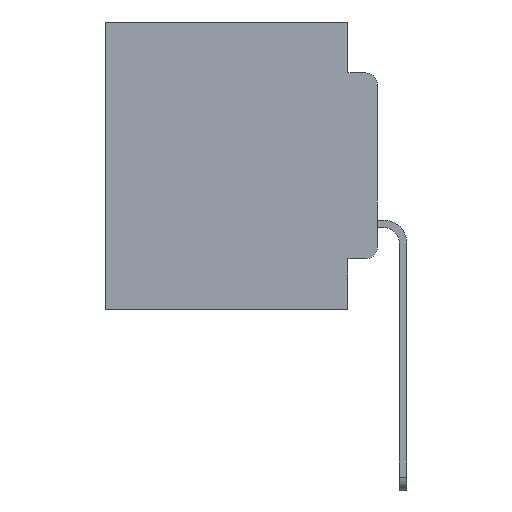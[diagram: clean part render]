
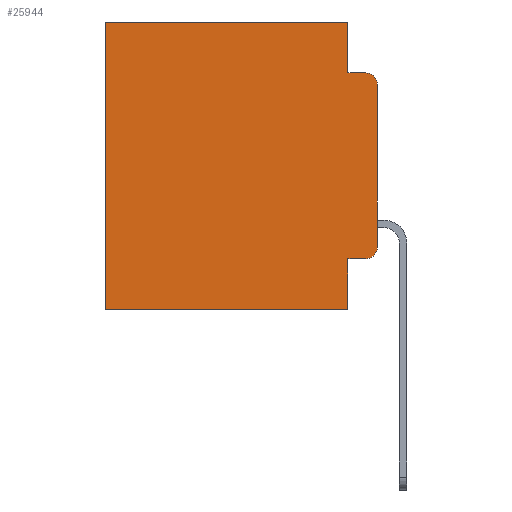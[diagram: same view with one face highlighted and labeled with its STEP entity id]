
A CAD part, left-side view. The second image highlights one B-rep face of the part: STEP entity #25944.
In plain terms, the highlighted planar face has unit normal (-1, 0, 0).
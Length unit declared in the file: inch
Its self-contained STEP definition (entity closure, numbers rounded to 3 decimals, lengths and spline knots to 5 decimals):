
#143 = CARTESIAN_POINT ( 'NONE',  ( 0.298, 0.051, 0. ) ) ;
#675 = EDGE_CURVE ( 'NONE', #21262, #17718, #24937, .T. ) ;
#770 = EDGE_CURVE ( 'NONE', #8905, #21262, #11966, .T. ) ;
#814 = EDGE_CURVE ( 'NONE', #8905, #18406, #3340, .T. ) ;
#872 = EDGE_CURVE ( 'NONE', #12851, #16531, #16743, .T. ) ;
#908 = EDGE_CURVE ( 'NONE', #21166, #15340, #10977, .T. ) ;
#920 = EDGE_CURVE ( 'NONE', #15340, #24086, #20566, .T. ) ;
#952 = EDGE_CURVE ( 'NONE', #9376, #24086, #14355, .T. ) ;
#1000 = EDGE_CURVE ( 'NONE', #9376, #17718, #1510, .T. ) ;
#1510 = LINE ( 'NONE', #13887, #7711 ) ;
#2971 = EDGE_CURVE ( 'NONE', #18406, #16531, #25428, .T. ) ;
#3140 = ORIENTED_EDGE ( 'NONE', *, *, #4649, .T. ) ;
#3340 = LINE ( 'NONE', #143, #10024 ) ;
#4429 = VECTOR ( 'NONE', #13042, 39.37008 ) ;
#4486 = CARTESIAN_POINT ( 'NONE',  ( 0.298, 0.051, -0.0885 ) ) ;
#4649 = EDGE_CURVE ( 'NONE', #21166, #12851, #20337, .T. ) ;
#5161 = AXIS2_PLACEMENT_3D ( 'NONE', #17156, #17014, #17749 ) ;
#5335 = ORIENTED_EDGE ( 'NONE', *, *, #675, .T. ) ;
#6407 = ORIENTED_EDGE ( 'NONE', *, *, #920, .F. ) ;
#6956 = PLANE ( 'NONE',  #23720 ) ;
#7711 = VECTOR ( 'NONE', #15707, 39.37008 ) ;
#8713 = DIRECTION ( 'NONE',  ( 0., 0., -1. ) ) ;
#8905 = VERTEX_POINT ( 'NONE', #20003 ) ;
#8941 = DIRECTION ( 'NONE',  ( 0., -1., 0. ) ) ;
#9144 = DIRECTION ( 'NONE',  ( 0., 0., -1. ) ) ;
#9376 = VERTEX_POINT ( 'NONE', #21919 ) ;
#9735 = CARTESIAN_POINT ( 'NONE',  ( 0.298, 0.473, -0.5 ) ) ;
#9826 = ORIENTED_EDGE ( 'NONE', *, *, #2971, .F. ) ;
#10024 = VECTOR ( 'NONE', #8713, 39.37008 ) ;
#10456 = ORIENTED_EDGE ( 'NONE', *, *, #770, .T. ) ;
#10885 = VECTOR ( 'NONE', #13957, 39.37008 ) ;
#10977 = LINE ( 'NONE', #17508, #25511 ) ;
#11966 = LINE ( 'NONE', #15348, #16449 ) ;
#12851 = VERTEX_POINT ( 'NONE', #17704 ) ;
#13042 = DIRECTION ( 'NONE',  ( 0., -1., 0. ) ) ;
#13094 = CARTESIAN_POINT ( 'NONE',  ( 0.298, 0.051, -0.0885 ) ) ;
#13291 = ORIENTED_EDGE ( 'NONE', *, *, #908, .F. ) ;
#13887 = CARTESIAN_POINT ( 'NONE',  ( 0.298, 0., 0. ) ) ;
#13957 = DIRECTION ( 'NONE',  ( 0., 1., 0. ) ) ;
#14355 = CIRCLE ( 'NONE', #22006, 0.02 ) ;
#15098 = ORIENTED_EDGE ( 'NONE', *, *, #814, .F. ) ;
#15340 = VERTEX_POINT ( 'NONE', #4486 ) ;
#15348 = CARTESIAN_POINT ( 'NONE',  ( 0.298, 0.051, -0.4115 ) ) ;
#15626 = CARTESIAN_POINT ( 'NONE',  ( 0.298, 0.473, 0. ) ) ;
#15707 = DIRECTION ( 'NONE',  ( 0., 0., -1. ) ) ;
#15964 = ORIENTED_EDGE ( 'NONE', *, *, #952, .T. ) ;
#16449 = VECTOR ( 'NONE', #8941, 39.37008 ) ;
#16531 = VERTEX_POINT ( 'NONE', #9735 ) ;
#16598 = DIRECTION ( 'NONE',  ( -1., 0., 0. ) ) ;
#16648 = CARTESIAN_POINT ( 'NONE',  ( 0.298, 0.02, -0.1085 ) ) ;
#16743 = LINE ( 'NONE', #15626, #22293 ) ;
#16797 = DIRECTION ( 'NONE',  ( 0., 0., -1. ) ) ;
#16883 = CARTESIAN_POINT ( 'NONE',  ( 0.298, 0.02, -0.0885 ) ) ;
#16969 = CARTESIAN_POINT ( 'NONE',  ( 0.298, 0., 0. ) ) ;
#17014 = DIRECTION ( 'NONE',  ( -1., 0., 0. ) ) ;
#17156 = CARTESIAN_POINT ( 'NONE',  ( 0.298, 0.02, -0.3915 ) ) ;
#17508 = CARTESIAN_POINT ( 'NONE',  ( 0.298, 0.051, 0. ) ) ;
#17540 = DIRECTION ( 'NONE',  ( 0., 0., -1. ) ) ;
#17704 = CARTESIAN_POINT ( 'NONE',  ( 0.298, 0.473, 0. ) ) ;
#17718 = VERTEX_POINT ( 'NONE', #19518 ) ;
#17749 = DIRECTION ( 'NONE',  ( 0., 0., -1. ) ) ;
#18406 = VERTEX_POINT ( 'NONE', #20817 ) ;
#19376 = DIRECTION ( 'NONE',  ( 0., 0., -1. ) ) ;
#19518 = CARTESIAN_POINT ( 'NONE',  ( 0.298, 0., -0.3915 ) ) ;
#20003 = CARTESIAN_POINT ( 'NONE',  ( 0.298, 0.051, -0.4115 ) ) ;
#20337 = LINE ( 'NONE', #22124, #24703 ) ;
#20376 = ORIENTED_EDGE ( 'NONE', *, *, #1000, .F. ) ;
#20566 = LINE ( 'NONE', #13094, #4429 ) ;
#20598 = DIRECTION ( 'NONE',  ( 0., 1., 0. ) ) ;
#20742 = DIRECTION ( 'NONE',  ( 1., 0., 0. ) ) ;
#20817 = CARTESIAN_POINT ( 'NONE',  ( 0.298, 0.051, -0.5 ) ) ;
#20820 = CARTESIAN_POINT ( 'NONE',  ( 0.298, 0.051, 0. ) ) ;
#21166 = VERTEX_POINT ( 'NONE', #20820 ) ;
#21262 = VERTEX_POINT ( 'NONE', #22829 ) ;
#21919 = CARTESIAN_POINT ( 'NONE',  ( 0.298, 0., -0.1085 ) ) ;
#22006 = AXIS2_PLACEMENT_3D ( 'NONE', #16648, #16598, #16797 ) ;
#22124 = CARTESIAN_POINT ( 'NONE',  ( 0.298, 0., 0. ) ) ;
#22293 = VECTOR ( 'NONE', #19376, 39.37008 ) ;
#22829 = CARTESIAN_POINT ( 'NONE',  ( 0.298, 0.02, -0.4115 ) ) ;
#23720 = AXIS2_PLACEMENT_3D ( 'NONE', #16969, #20742, #9144 ) ;
#24086 = VERTEX_POINT ( 'NONE', #16883 ) ;
#24199 = EDGE_LOOP ( 'NONE', ( #20376, #15964, #6407, #13291, #3140, #24467, #9826, #15098, #10456, #5335 ) ) ;
#24467 = ORIENTED_EDGE ( 'NONE', *, *, #872, .T. ) ;
#24703 = VECTOR ( 'NONE', #20598, 39.37008 ) ;
#24937 = CIRCLE ( 'NONE', #5161, 0.02 ) ;
#25345 = CARTESIAN_POINT ( 'NONE',  ( 0.298, 0., -0.5 ) ) ;
#25428 = LINE ( 'NONE', #25345, #10885 ) ;
#25511 = VECTOR ( 'NONE', #17540, 39.37008 ) ;
#25641 = FACE_OUTER_BOUND ( 'NONE', #24199, .T. ) ;
#25944 = ADVANCED_FACE ( 'NONE', ( #25641 ), #6956, .F. ) ;
